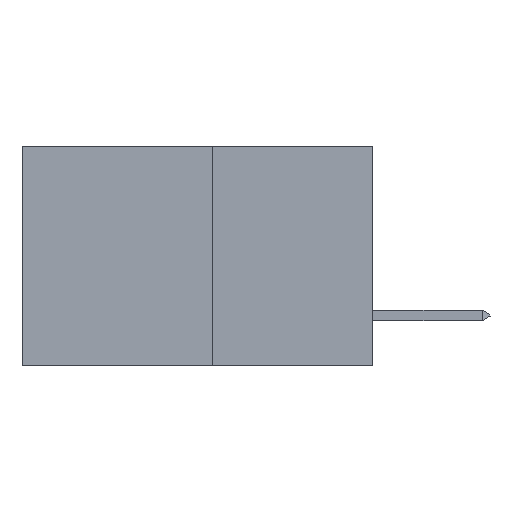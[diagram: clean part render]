
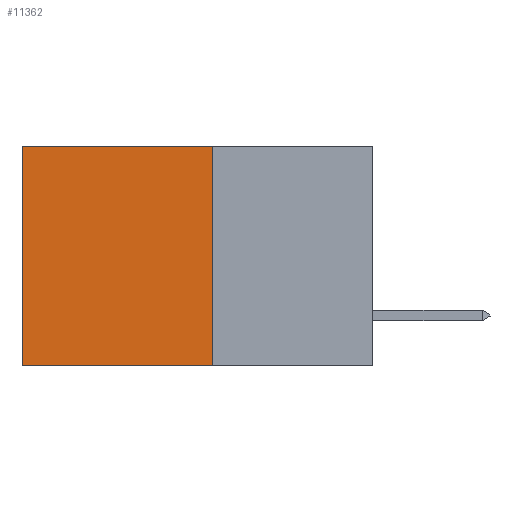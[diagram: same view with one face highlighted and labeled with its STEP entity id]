
A CAD part, left-side view. The second image highlights one B-rep face of the part: STEP entity #11362.
In plain terms, the highlighted planar face has unit normal (-1, 0, 0).
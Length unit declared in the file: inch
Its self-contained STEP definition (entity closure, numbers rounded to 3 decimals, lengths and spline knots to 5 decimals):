
#1079 = VECTOR ( 'NONE', #17442, 39.37008 ) ;
#1500 = EDGE_CURVE ( 'NONE', #7883, #14516, #18355, .T. ) ;
#1746 = ORIENTED_EDGE ( 'NONE', *, *, #1500, .T. ) ;
#3264 = EDGE_CURVE ( 'NONE', #14516, #16436, #11855, .T. ) ;
#3547 = CARTESIAN_POINT ( 'NONE',  ( 0.277, 0.27, -0.37 ) ) ;
#3775 = ORIENTED_EDGE ( 'NONE', *, *, #3264, .T. ) ;
#4138 = LINE ( 'NONE', #3547, #16605 ) ;
#5036 = CARTESIAN_POINT ( 'NONE',  ( 0.277, 0.59, 0. ) ) ;
#6547 = DIRECTION ( 'NONE',  ( 0., 0., -1. ) ) ;
#6952 = CARTESIAN_POINT ( 'NONE',  ( 0.277, 0.27, -0.37 ) ) ;
#6996 = VERTEX_POINT ( 'NONE', #6952 ) ;
#7024 = PLANE ( 'NONE',  #10077 ) ;
#7187 = ORIENTED_EDGE ( 'NONE', *, *, #15791, .F. ) ;
#7401 = EDGE_CURVE ( 'NONE', #6996, #16436, #4138, .T. ) ;
#7403 = CARTESIAN_POINT ( 'NONE',  ( 0.277, 0.27, -0.37 ) ) ;
#7637 = EDGE_LOOP ( 'NONE', ( #3775, #11732, #7187, #1746 ) ) ;
#7883 = VERTEX_POINT ( 'NONE', #10497 ) ;
#7979 = VECTOR ( 'NONE', #6547, 39.37008 ) ;
#8386 = LINE ( 'NONE', #7403, #1079 ) ;
#9959 = DIRECTION ( 'NONE',  ( 0., 0., -1. ) ) ;
#10077 = AXIS2_PLACEMENT_3D ( 'NONE', #17086, #18496, #9959 ) ;
#10497 = CARTESIAN_POINT ( 'NONE',  ( 0.277, 0.27, 0. ) ) ;
#10782 = VECTOR ( 'NONE', #13919, 39.37008 ) ;
#11362 = ADVANCED_FACE ( 'NONE', ( #16689 ), #7024, .F. ) ;
#11732 = ORIENTED_EDGE ( 'NONE', *, *, #7401, .F. ) ;
#11855 = LINE ( 'NONE', #11874, #7979 ) ;
#11874 = CARTESIAN_POINT ( 'NONE',  ( 0.277, 0.59, -0.37 ) ) ;
#13685 = DIRECTION ( 'NONE',  ( 0., 1., 0. ) ) ;
#13919 = DIRECTION ( 'NONE',  ( 0., 1., 0. ) ) ;
#14516 = VERTEX_POINT ( 'NONE', #5036 ) ;
#14567 = CARTESIAN_POINT ( 'NONE',  ( 0.277, 0.27, 0. ) ) ;
#14617 = CARTESIAN_POINT ( 'NONE',  ( 0.277, 0.59, -0.37 ) ) ;
#15791 = EDGE_CURVE ( 'NONE', #7883, #6996, #8386, .T. ) ;
#16436 = VERTEX_POINT ( 'NONE', #14617 ) ;
#16605 = VECTOR ( 'NONE', #13685, 39.37008 ) ;
#16689 = FACE_OUTER_BOUND ( 'NONE', #7637, .T. ) ;
#17086 = CARTESIAN_POINT ( 'NONE',  ( 0.277, 0.27, -0.37 ) ) ;
#17442 = DIRECTION ( 'NONE',  ( 0., 0., -1. ) ) ;
#18355 = LINE ( 'NONE', #14567, #10782 ) ;
#18496 = DIRECTION ( 'NONE',  ( 1., 0., 0. ) ) ;
